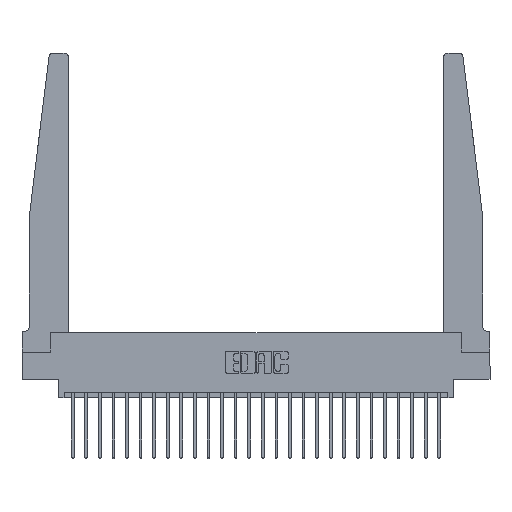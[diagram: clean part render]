
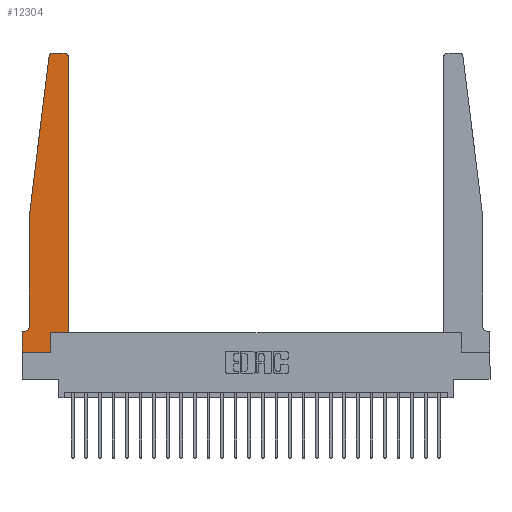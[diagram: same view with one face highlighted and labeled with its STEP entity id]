
A CAD part, top view. The second image highlights one B-rep face of the part: STEP entity #12304.
In plain terms, the highlighted planar face has unit normal (0, 0, 1).
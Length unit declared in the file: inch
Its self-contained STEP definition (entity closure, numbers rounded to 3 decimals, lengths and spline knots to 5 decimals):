
#48 = CARTESIAN_POINT ( 'NONE',  ( 0.395, 2.75, 0.37 ) ) ;
#106 = CARTESIAN_POINT ( 'NONE',  ( 0.425, 0.18, 0.37 ) ) ;
#230 = VECTOR ( 'NONE', #25066, 39.37008 ) ;
#331 = DIRECTION ( 'NONE',  ( 1., 0., 0. ) ) ;
#675 = CARTESIAN_POINT ( 'NONE',  ( 0.24675, 2.72367, 0.37 ) ) ;
#842 = LINE ( 'NONE', #13564, #230 ) ;
#850 = VECTOR ( 'NONE', #1582, 39.37008 ) ;
#1304 = CARTESIAN_POINT ( 'NONE',  ( 0.27653, 2.72, 0.37 ) ) ;
#1357 = EDGE_CURVE ( 'NONE', #20451, #22613, #1711, .T. ) ;
#1582 = DIRECTION ( 'NONE',  ( -0.122, -0.992, 0. ) ) ;
#1595 = CARTESIAN_POINT ( 'NONE',  ( 0.25, 2.75, 0.37 ) ) ;
#1604 = ORIENTED_EDGE ( 'NONE', *, *, #3201, .T. ) ;
#1711 = LINE ( 'NONE', #14200, #21154 ) ;
#1727 = VERTEX_POINT ( 'NONE', #17220 ) ;
#3201 = EDGE_CURVE ( 'NONE', #15033, #9778, #16738, .T. ) ;
#3214 = AXIS2_PLACEMENT_3D ( 'NONE', #22080, #10520, #24012 ) ;
#3276 = DIRECTION ( 'NONE',  ( 1., 0., 0. ) ) ;
#3314 = VECTOR ( 'NONE', #8124, 39.37008 ) ;
#4446 = DIRECTION ( 'NONE',  ( 0., 1., 0. ) ) ;
#4583 = VECTOR ( 'NONE', #24803, 39.37008 ) ;
#4592 = VECTOR ( 'NONE', #7132, 39.37008 ) ;
#4737 = AXIS2_PLACEMENT_3D ( 'NONE', #5196, #18815, #7156 ) ;
#4934 = CARTESIAN_POINT ( 'NONE',  ( 0.065, 0.2375, 0.37 ) ) ;
#5099 = CARTESIAN_POINT ( 'NONE',  ( 0.2605, 0.18, 0.37 ) ) ;
#5196 = CARTESIAN_POINT ( 'NONE',  ( 0.395, 2.72, 0.37 ) ) ;
#5461 = DIRECTION ( 'NONE',  ( 1., 0., 0. ) ) ;
#5466 = CARTESIAN_POINT ( 'NONE',  ( 0.015, 0.1875, 0.37 ) ) ;
#5757 = ORIENTED_EDGE ( 'NONE', *, *, #24444, .T. ) ;
#6041 = LINE ( 'NONE', #9357, #850 ) ;
#6607 = EDGE_CURVE ( 'NONE', #8809, #20451, #15360, .T. ) ;
#6612 = LINE ( 'NONE', #17475, #11178 ) ;
#7132 = DIRECTION ( 'NONE',  ( 0., 1., 0. ) ) ;
#7156 = DIRECTION ( 'NONE',  ( 1., 0., 0. ) ) ;
#7260 = CARTESIAN_POINT ( 'NONE',  ( 0., 0., 0.37 ) ) ;
#7357 = VERTEX_POINT ( 'NONE', #48 ) ;
#7905 = ORIENTED_EDGE ( 'NONE', *, *, #19234, .T. ) ;
#7938 = FACE_OUTER_BOUND ( 'NONE', #17891, .T. ) ;
#8124 = DIRECTION ( 'NONE',  ( 0., -1., 0. ) ) ;
#8416 = EDGE_CURVE ( 'NONE', #23807, #11383, #6612, .T. ) ;
#8809 = VERTEX_POINT ( 'NONE', #5099 ) ;
#8824 = CARTESIAN_POINT ( 'NONE',  ( 0., 0.1875, 0.37 ) ) ;
#8945 = VERTEX_POINT ( 'NONE', #17842 ) ;
#9357 = CARTESIAN_POINT ( 'NONE',  ( 0.065, 1.25, 0.37 ) ) ;
#9778 = VERTEX_POINT ( 'NONE', #675 ) ;
#9795 = LINE ( 'NONE', #16824, #4592 ) ;
#9859 = VERTEX_POINT ( 'NONE', #4934 ) ;
#10337 = AXIS2_PLACEMENT_3D ( 'NONE', #8824, #24269, #12743 ) ;
#10392 = LINE ( 'NONE', #1595, #4583 ) ;
#10520 = DIRECTION ( 'NONE',  ( 0., 0., -1. ) ) ;
#10652 = CARTESIAN_POINT ( 'NONE',  ( 0.425, 2.72, 0.37 ) ) ;
#11178 = VECTOR ( 'NONE', #19410, 39.37008 ) ;
#11383 = VERTEX_POINT ( 'NONE', #21063 ) ;
#12304 = ADVANCED_FACE ( 'NONE', ( #7938 ), #20420, .T. ) ;
#12743 = DIRECTION ( 'NONE',  ( 1., 0., 0. ) ) ;
#12748 = ORIENTED_EDGE ( 'NONE', *, *, #1357, .T. ) ;
#13001 = VERTEX_POINT ( 'NONE', #7260 ) ;
#13028 = CIRCLE ( 'NONE', #4737, 0.03 ) ;
#13197 = CIRCLE ( 'NONE', #3214, 0.05 ) ;
#13564 = CARTESIAN_POINT ( 'NONE',  ( 0.065, 1.25, 0.37 ) ) ;
#13638 = ORIENTED_EDGE ( 'NONE', *, *, #18641, .T. ) ;
#14200 = CARTESIAN_POINT ( 'NONE',  ( 0.425, 0.18, 0.37 ) ) ;
#14783 = AXIS2_PLACEMENT_3D ( 'NONE', #1304, #14956, #3276 ) ;
#14956 = DIRECTION ( 'NONE',  ( 0., 0., 1. ) ) ;
#14961 = EDGE_CURVE ( 'NONE', #22613, #7357, #13028, .T. ) ;
#14962 = ORIENTED_EDGE ( 'NONE', *, *, #24009, .T. ) ;
#15033 = VERTEX_POINT ( 'NONE', #17026 ) ;
#15360 = LINE ( 'NONE', #24819, #21074 ) ;
#16074 = ORIENTED_EDGE ( 'NONE', *, *, #17191, .T. ) ;
#16689 = ORIENTED_EDGE ( 'NONE', *, *, #8416, .T. ) ;
#16738 = CIRCLE ( 'NONE', #14783, 0.03 ) ;
#16824 = CARTESIAN_POINT ( 'NONE',  ( 0.2605, 0.18, 0.37 ) ) ;
#17026 = CARTESIAN_POINT ( 'NONE',  ( 0.27653, 2.75, 0.37 ) ) ;
#17191 = EDGE_CURVE ( 'NONE', #1727, #8809, #9795, .T. ) ;
#17220 = CARTESIAN_POINT ( 'NONE',  ( 0.2605, 0., 0.37 ) ) ;
#17332 = ORIENTED_EDGE ( 'NONE', *, *, #14961, .T. ) ;
#17475 = CARTESIAN_POINT ( 'NONE',  ( 0.065, 0.1875, 0.37 ) ) ;
#17558 = ORIENTED_EDGE ( 'NONE', *, *, #21934, .T. ) ;
#17842 = CARTESIAN_POINT ( 'NONE',  ( 0.065, 1.25, 0.37 ) ) ;
#17891 = EDGE_LOOP ( 'NONE', ( #23824, #1604, #5757, #7905, #17558, #16689, #13638, #14962, #16074, #19457, #12748, #17332 ) ) ;
#18641 = EDGE_CURVE ( 'NONE', #11383, #13001, #20052, .T. ) ;
#18815 = DIRECTION ( 'NONE',  ( 0., 0., 1. ) ) ;
#19234 = EDGE_CURVE ( 'NONE', #8945, #9859, #842, .T. ) ;
#19410 = DIRECTION ( 'NONE',  ( -1., 0., 0. ) ) ;
#19457 = ORIENTED_EDGE ( 'NONE', *, *, #6607, .T. ) ;
#20052 = LINE ( 'NONE', #21636, #3314 ) ;
#20334 = LINE ( 'NONE', #23651, #21521 ) ;
#20420 = PLANE ( 'NONE',  #10337 ) ;
#20451 = VERTEX_POINT ( 'NONE', #106 ) ;
#21063 = CARTESIAN_POINT ( 'NONE',  ( 0., 0.1875, 0.37 ) ) ;
#21074 = VECTOR ( 'NONE', #5461, 39.37008 ) ;
#21154 = VECTOR ( 'NONE', #4446, 39.37008 ) ;
#21521 = VECTOR ( 'NONE', #331, 39.37008 ) ;
#21636 = CARTESIAN_POINT ( 'NONE',  ( 0., 0., 0.37 ) ) ;
#21934 = EDGE_CURVE ( 'NONE', #9859, #23807, #13197, .T. ) ;
#22080 = CARTESIAN_POINT ( 'NONE',  ( 0.015, 0.2375, 0.37 ) ) ;
#22613 = VERTEX_POINT ( 'NONE', #10652 ) ;
#22834 = EDGE_CURVE ( 'NONE', #7357, #15033, #10392, .T. ) ;
#23651 = CARTESIAN_POINT ( 'NONE',  ( 0., 0., 0.37 ) ) ;
#23807 = VERTEX_POINT ( 'NONE', #5466 ) ;
#23824 = ORIENTED_EDGE ( 'NONE', *, *, #22834, .T. ) ;
#24009 = EDGE_CURVE ( 'NONE', #13001, #1727, #20334, .T. ) ;
#24012 = DIRECTION ( 'NONE',  ( -1., 0., 0. ) ) ;
#24269 = DIRECTION ( 'NONE',  ( 0., 0., 1. ) ) ;
#24444 = EDGE_CURVE ( 'NONE', #9778, #8945, #6041, .T. ) ;
#24803 = DIRECTION ( 'NONE',  ( -1., 0., 0. ) ) ;
#24819 = CARTESIAN_POINT ( 'NONE',  ( 0.425, 0.18, 0.37 ) ) ;
#25066 = DIRECTION ( 'NONE',  ( 0., -1., 0. ) ) ;
